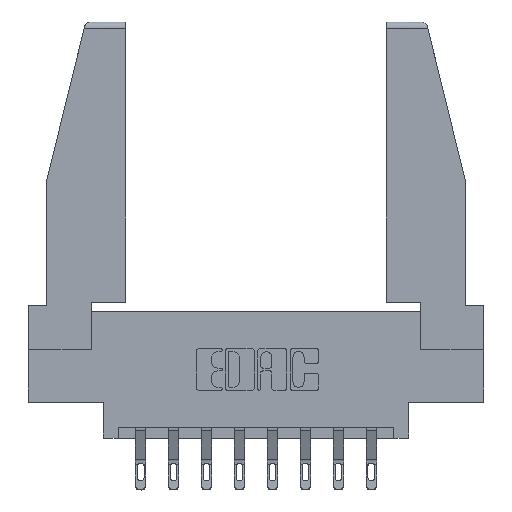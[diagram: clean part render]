
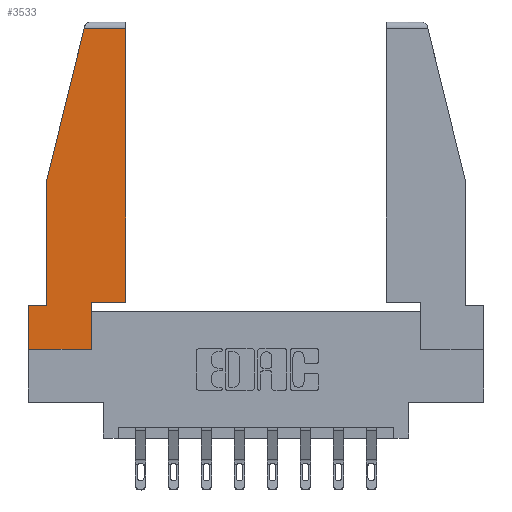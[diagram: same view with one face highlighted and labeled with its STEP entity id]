
A CAD part, top view. The second image highlights one B-rep face of the part: STEP entity #3533.
In plain terms, the highlighted planar face has unit normal (0, 0, 1).
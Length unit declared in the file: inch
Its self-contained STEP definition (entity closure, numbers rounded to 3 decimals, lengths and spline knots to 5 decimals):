
#28 = PLANE ( 'NONE',  #11604 ) ;
#178 = CARTESIAN_POINT ( 'NONE',  ( 0.086, 0.8, 0. ) ) ;
#414 = VECTOR ( 'NONE', #9575, 39.37008 ) ;
#446 = ORIENTED_EDGE ( 'NONE', *, *, #6288, .T. ) ;
#726 = CARTESIAN_POINT ( 'NONE',  ( 0., 0.21, 0. ) ) ;
#754 = CARTESIAN_POINT ( 'NONE',  ( 0., 0., 0. ) ) ;
#930 = DIRECTION ( 'NONE',  ( 0., 0., 1. ) ) ;
#1065 = CARTESIAN_POINT ( 'NONE',  ( 0., 0., 0. ) ) ;
#1307 = DIRECTION ( 'NONE',  ( 0., -1., 0. ) ) ;
#1450 = CARTESIAN_POINT ( 'NONE',  ( 0.461, 0.223, 0. ) ) ;
#2097 = DIRECTION ( 'NONE',  ( 1., 0., 0. ) ) ;
#2120 = VERTEX_POINT ( 'NONE', #4496 ) ;
#2979 = VECTOR ( 'NONE', #6210, 39.37008 ) ;
#3089 = CARTESIAN_POINT ( 'NONE',  ( 0.297, 0., 0. ) ) ;
#3106 = ORIENTED_EDGE ( 'NONE', *, *, #6020, .T. ) ;
#3180 = VECTOR ( 'NONE', #8345, 39.37008 ) ;
#3252 = VERTEX_POINT ( 'NONE', #4545 ) ;
#3533 = ADVANCED_FACE ( 'NONE', ( #5697 ), #28, .T. ) ;
#4037 = LINE ( 'NONE', #10805, #11082 ) ;
#4105 = CARTESIAN_POINT ( 'NONE',  ( 0.086, 0.8, 0. ) ) ;
#4496 = CARTESIAN_POINT ( 'NONE',  ( 0.461, 1.52, 0. ) ) ;
#4545 = CARTESIAN_POINT ( 'NONE',  ( 0.086, 0.21, 0. ) ) ;
#4630 = LINE ( 'NONE', #5306, #414 ) ;
#4759 = LINE ( 'NONE', #754, #13125 ) ;
#4895 = EDGE_CURVE ( 'NONE', #9959, #2120, #12865, .T. ) ;
#5065 = CARTESIAN_POINT ( 'NONE',  ( 0.297, 0., 0. ) ) ;
#5077 = DIRECTION ( 'NONE',  ( -1., 0., 0. ) ) ;
#5273 = VERTEX_POINT ( 'NONE', #6476 ) ;
#5306 = CARTESIAN_POINT ( 'NONE',  ( 0., 0.21, 0. ) ) ;
#5697 = FACE_OUTER_BOUND ( 'NONE', #8285, .T. ) ;
#5728 = ORIENTED_EDGE ( 'NONE', *, *, #7571, .T. ) ;
#6005 = DIRECTION ( 'NONE',  ( 1., 0., 0. ) ) ;
#6008 = LINE ( 'NONE', #5065, #3180 ) ;
#6020 = EDGE_CURVE ( 'NONE', #12193, #9461, #9054, .T. ) ;
#6210 = DIRECTION ( 'NONE',  ( -1., 0., 0. ) ) ;
#6274 = CARTESIAN_POINT ( 'NONE',  ( 0.461, 0.223, 0. ) ) ;
#6288 = EDGE_CURVE ( 'NONE', #9461, #3252, #11852, .T. ) ;
#6476 = CARTESIAN_POINT ( 'NONE',  ( 0., 0., 0. ) ) ;
#6622 = VECTOR ( 'NONE', #10066, 39.37008 ) ;
#6912 = ORIENTED_EDGE ( 'NONE', *, *, #8713, .T. ) ;
#6946 = ORIENTED_EDGE ( 'NONE', *, *, #11311, .T. ) ;
#7447 = ORIENTED_EDGE ( 'NONE', *, *, #4895, .T. ) ;
#7571 = EDGE_CURVE ( 'NONE', #5273, #10135, #4759, .T. ) ;
#7634 = VECTOR ( 'NONE', #9360, 39.37008 ) ;
#7642 = CARTESIAN_POINT ( 'NONE',  ( 0.2636, 1.52, 0. ) ) ;
#7920 = VECTOR ( 'NONE', #1307, 39.37008 ) ;
#8285 = EDGE_LOOP ( 'NONE', ( #7447, #9269, #3106, #446, #12270, #6946, #5728, #6912, #8740 ) ) ;
#8345 = DIRECTION ( 'NONE',  ( 0., 1., 0. ) ) ;
#8713 = EDGE_CURVE ( 'NONE', #10135, #9220, #6008, .T. ) ;
#8728 = DIRECTION ( 'NONE',  ( 1., 0., 0. ) ) ;
#8740 = ORIENTED_EDGE ( 'NONE', *, *, #9150, .T. ) ;
#9016 = LINE ( 'NONE', #11361, #9517 ) ;
#9054 = LINE ( 'NONE', #9760, #6622 ) ;
#9056 = CARTESIAN_POINT ( 'NONE',  ( 0., 0.21, 0. ) ) ;
#9150 = EDGE_CURVE ( 'NONE', #9220, #9959, #4037, .T. ) ;
#9220 = VERTEX_POINT ( 'NONE', #12952 ) ;
#9269 = ORIENTED_EDGE ( 'NONE', *, *, #12345, .T. ) ;
#9360 = DIRECTION ( 'NONE',  ( 0., 1., 0. ) ) ;
#9461 = VERTEX_POINT ( 'NONE', #4105 ) ;
#9517 = VECTOR ( 'NONE', #5077, 39.37008 ) ;
#9575 = DIRECTION ( 'NONE',  ( 0., -1., 0. ) ) ;
#9760 = CARTESIAN_POINT ( 'NONE',  ( 0.271, 1.55, 0. ) ) ;
#9959 = VERTEX_POINT ( 'NONE', #1450 ) ;
#10066 = DIRECTION ( 'NONE',  ( -0.239, -0.971, 0. ) ) ;
#10135 = VERTEX_POINT ( 'NONE', #3089 ) ;
#10740 = VERTEX_POINT ( 'NONE', #9056 ) ;
#10805 = CARTESIAN_POINT ( 'NONE',  ( 0.297, 0.223, 0. ) ) ;
#11082 = VECTOR ( 'NONE', #8728, 39.37008 ) ;
#11311 = EDGE_CURVE ( 'NONE', #10740, #5273, #4630, .T. ) ;
#11361 = CARTESIAN_POINT ( 'NONE',  ( 0., 1.52, 0. ) ) ;
#11364 = EDGE_CURVE ( 'NONE', #3252, #10740, #13307, .T. ) ;
#11604 = AXIS2_PLACEMENT_3D ( 'NONE', #1065, #930, #2097 ) ;
#11852 = LINE ( 'NONE', #178, #7920 ) ;
#12193 = VERTEX_POINT ( 'NONE', #7642 ) ;
#12270 = ORIENTED_EDGE ( 'NONE', *, *, #11364, .T. ) ;
#12345 = EDGE_CURVE ( 'NONE', #2120, #12193, #9016, .T. ) ;
#12865 = LINE ( 'NONE', #6274, #7634 ) ;
#12952 = CARTESIAN_POINT ( 'NONE',  ( 0.297, 0.223, 0. ) ) ;
#13125 = VECTOR ( 'NONE', #6005, 39.37008 ) ;
#13307 = LINE ( 'NONE', #726, #2979 ) ;
